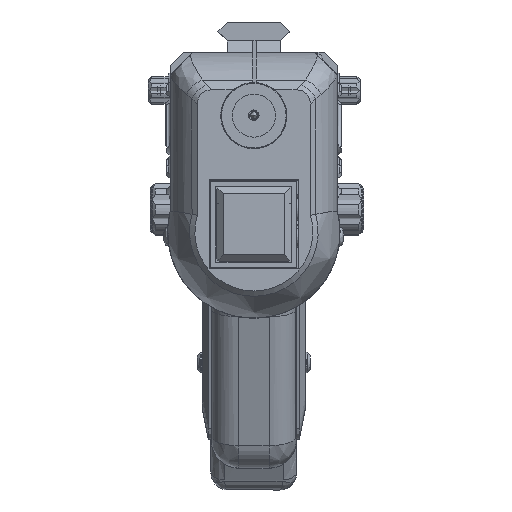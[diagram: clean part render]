
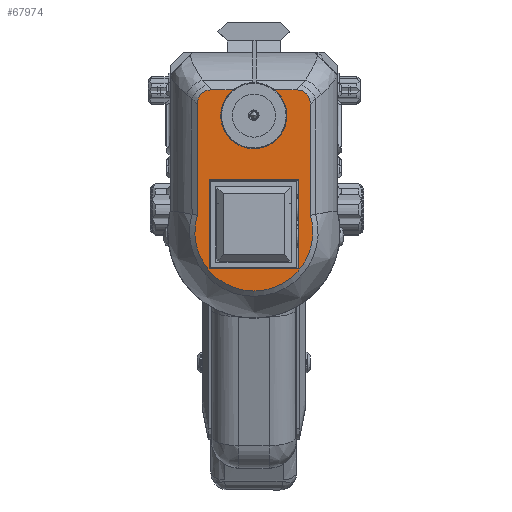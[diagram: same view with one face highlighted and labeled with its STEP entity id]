
A CAD part, left-side view. The second image highlights one B-rep face of the part: STEP entity #67974.
In plain terms, the highlighted planar face has unit normal (-1, 0, 0).
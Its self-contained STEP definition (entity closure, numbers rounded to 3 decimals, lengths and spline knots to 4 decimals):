
#581=ELLIPSE($,#72353,1.0392,0.6);
#582=ELLIPSE($,#72354,1.0392,0.6);
#2598=LINE($,#96876,#8961);
#2601=LINE($,#96881,#8964);
#2603=LINE($,#96889,#8966);
#2605=LINE($,#96892,#8968);
#2609=LINE($,#97083,#8972);
#2610=LINE($,#97085,#8973);
#2611=LINE($,#97089,#8974);
#2612=LINE($,#97092,#8975);
#8961=VECTOR($,#78494,2.6402);
#8964=VECTOR($,#78499,2.64);
#8966=VECTOR($,#78507,2.6402);
#8968=VECTOR($,#78511,2.64);
#8972=VECTOR($,#78577,3.2737);
#8973=VECTOR($,#78578,3.2737);
#8974=VECTOR($,#78581,0.6386);
#8975=VECTOR($,#78584,0.6386);
#16298=FACE_BOUND($,#21798,.T.);
#17805=FACE_OUTER_BOUND($,#21797,.T.);
#21797=EDGE_LOOP($,(#45947,#45948,#45949,#45950,#45951,#45952,#45953,#45954));
#21798=EDGE_LOOP($,(#45955,#45956,#45957,#45958));
#27148=CIRCLE($,#72314,1.74);
#27166=CIRCLE($,#72355,0.975);
#28990=VERTEX_POINT($,#96858);
#28991=VERTEX_POINT($,#96863);
#28994=VERTEX_POINT($,#96874);
#28995=VERTEX_POINT($,#96875);
#28996=VERTEX_POINT($,#96880);
#28999=VERTEX_POINT($,#96888);
#29018=VERTEX_POINT($,#97080);
#29019=VERTEX_POINT($,#97081);
#29020=VERTEX_POINT($,#97084);
#29021=VERTEX_POINT($,#97086);
#29022=VERTEX_POINT($,#97088);
#29023=VERTEX_POINT($,#97090);
#35866=EDGE_CURVE($,#28990,#28991,#27148,.T.);
#35870=EDGE_CURVE($,#28994,#28995,#2598,.T.);
#35873=EDGE_CURVE($,#28994,#28996,#2601,.T.);
#35877=EDGE_CURVE($,#28999,#28996,#2603,.T.);
#35879=EDGE_CURVE($,#28995,#28999,#2605,.T.);
#35900=EDGE_CURVE($,#29018,#29019,#581,.T.);
#35901=EDGE_CURVE($,#28991,#29018,#2609,.T.);
#35902=EDGE_CURVE($,#29020,#28990,#2610,.T.);
#35903=EDGE_CURVE($,#29021,#29020,#582,.T.);
#35904=EDGE_CURVE($,#29022,#29021,#2611,.F.);
#35905=EDGE_CURVE($,#29022,#29023,#27166,.T.);
#35906=EDGE_CURVE($,#29019,#29023,#2612,.F.);
#45947=ORIENTED_EDGE($,*,*,#35900,.F.);
#45948=ORIENTED_EDGE($,*,*,#35901,.F.);
#45949=ORIENTED_EDGE($,*,*,#35866,.F.);
#45950=ORIENTED_EDGE($,*,*,#35902,.F.);
#45951=ORIENTED_EDGE($,*,*,#35903,.F.);
#45952=ORIENTED_EDGE($,*,*,#35904,.F.);
#45953=ORIENTED_EDGE($,*,*,#35905,.T.);
#45954=ORIENTED_EDGE($,*,*,#35906,.F.);
#45955=ORIENTED_EDGE($,*,*,#35870,.T.);
#45956=ORIENTED_EDGE($,*,*,#35879,.T.);
#45957=ORIENTED_EDGE($,*,*,#35877,.T.);
#45958=ORIENTED_EDGE($,*,*,#35873,.F.);
#65476=PLANE($,#72352);
#67974=ADVANCED_FACE($,(#17805,#16298),#65476,.F.);
#72314=AXIS2_PLACEMENT_3D($,#96864,#78486,#78487);
#72352=AXIS2_PLACEMENT_3D($,#97079,#78573,#78574);
#72353=AXIS2_PLACEMENT_3D($,#97082,#78575,#78576);
#72354=AXIS2_PLACEMENT_3D($,#97087,#78579,#78580);
#72355=AXIS2_PLACEMENT_3D($,#97091,#78582,#78583);
#78486=DIRECTION('center_axis',(1.,0.,0.));
#78487=DIRECTION('ref_axis',(0.,0.,-1.));
#78494=DIRECTION($,(0.,0.,1.));
#78499=DIRECTION($,(0.,-1.,0.));
#78507=DIRECTION($,(0.,0.,-1.));
#78511=DIRECTION($,(0.,-1.,0.));
#78573=DIRECTION('center_axis',(1.,0.,0.));
#78574=DIRECTION('ref_axis',(0.,0.,-1.));
#78575=DIRECTION('center_axis',(1.,0.,0.));
#78576=DIRECTION('ref_axis',(0.,0.707,0.707));
#78577=DIRECTION($,(0.,0.,1.));
#78578=DIRECTION($,(0.,0.,-1.));
#78579=DIRECTION('center_axis',(1.,0.,0.));
#78580=DIRECTION('ref_axis',(0.,-0.707,
0.707));
#78581=DIRECTION($,(0.,1.,0.));
#78582=DIRECTION('center_axis',(1.,0.,0.));
#78583=DIRECTION('ref_axis',(0.,0.,-1.));
#78584=DIRECTION($,(0.,1.,0.));
#96858=CARTESIAN_POINT('',(1.17,5.8319,8.2649));
#96863=CARTESIAN_POINT('',(1.17,9.1681,8.2649));
#96864=CARTESIAN_POINT('Origin',(1.17,7.5,7.7698));
#96874=CARTESIAN_POINT('',(1.17,8.82,6.6798));
#96875=CARTESIAN_POINT('',(1.17,8.82,9.32));
#96876=CARTESIAN_POINT($,(1.17,8.82,8.115));
#96880=CARTESIAN_POINT('',(1.17,6.18,6.6798));
#96881=CARTESIAN_POINT($,(1.17,7.4111,6.6798));
#96888=CARTESIAN_POINT('',(1.17,6.18,9.32));
#96889=CARTESIAN_POINT($,(1.17,6.18,9.385));
#96892=CARTESIAN_POINT($,(1.17,8.135,9.32));
#97079=CARTESIAN_POINT('Origin',(1.17,7.5,9.5));
#97080=CARTESIAN_POINT('',(1.17,9.17,11.5386));
#97081=CARTESIAN_POINT('',(1.17,8.7457,11.9629));
#97082=CARTESIAN_POINT('Origin',(1.17,8.3215,11.1144));
#97083=CARTESIAN_POINT($,(1.17,9.17,8.115));
#97084=CARTESIAN_POINT('',(1.17,5.83,11.5386));
#97085=CARTESIAN_POINT($,(1.17,5.83,9.385));
#97086=CARTESIAN_POINT('',(1.17,6.2543,11.9629));
#97087=CARTESIAN_POINT('Origin',(1.17,6.6785,11.1144));
#97088=CARTESIAN_POINT('',(1.17,6.8929,11.9629));
#97089=CARTESIAN_POINT($,(1.17,7.8175,11.9629));
#97090=CARTESIAN_POINT('',(1.17,8.1071,11.9629));
#97091=CARTESIAN_POINT('Origin',(1.17,7.5,11.2));
#97092=CARTESIAN_POINT($,(1.17,7.8175,11.9629));
